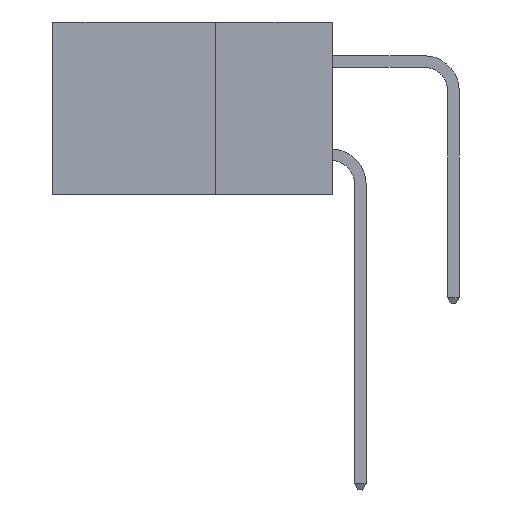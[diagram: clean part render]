
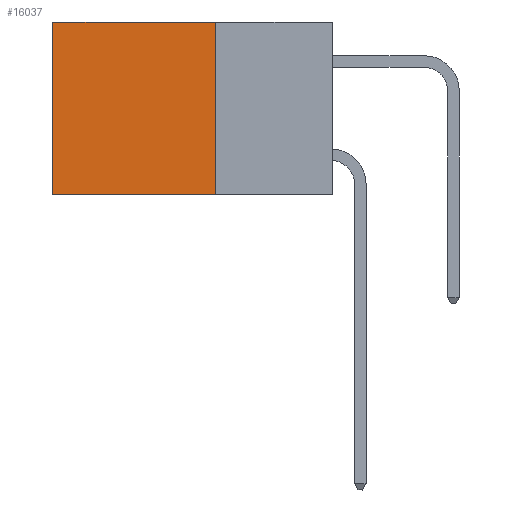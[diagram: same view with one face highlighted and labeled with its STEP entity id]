
A CAD part, left-side view. The second image highlights one B-rep face of the part: STEP entity #16037.
In plain terms, the highlighted planar face has unit normal (-1, 0, 0).
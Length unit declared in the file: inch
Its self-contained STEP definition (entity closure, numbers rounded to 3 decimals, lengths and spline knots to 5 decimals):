
#307 = ORIENTED_EDGE ( 'NONE', *, *, #5487, .T. ) ;
#901 = PLANE ( 'NONE',  #30332 ) ;
#1671 = CARTESIAN_POINT ( 'NONE',  ( 0.298, 0.6, 0. ) ) ;
#4353 = FACE_OUTER_BOUND ( 'NONE', #22903, .T. ) ;
#4789 = VECTOR ( 'NONE', #14758, 39.37008 ) ;
#5099 = VERTEX_POINT ( 'NONE', #7915 ) ;
#5487 = EDGE_CURVE ( 'NONE', #5099, #25406, #22364, .T. ) ;
#6231 = VECTOR ( 'NONE', #30755, 39.37008 ) ;
#6357 = DIRECTION ( 'NONE',  ( 0., 0., -1. ) ) ;
#6501 = CARTESIAN_POINT ( 'NONE',  ( 0.298, 0.25, 0. ) ) ;
#7915 = CARTESIAN_POINT ( 'NONE',  ( 0.298, 0.6, 0. ) ) ;
#8880 = EDGE_CURVE ( 'NONE', #11142, #5099, #28286, .T. ) ;
#9814 = ORIENTED_EDGE ( 'NONE', *, *, #23016, .F. ) ;
#10846 = VERTEX_POINT ( 'NONE', #28779 ) ;
#11142 = VERTEX_POINT ( 'NONE', #16438 ) ;
#11701 = CARTESIAN_POINT ( 'NONE',  ( 0.298, 0.25, 0. ) ) ;
#13079 = VECTOR ( 'NONE', #28653, 39.37008 ) ;
#14372 = VECTOR ( 'NONE', #18755, 39.37008 ) ;
#14758 = DIRECTION ( 'NONE',  ( 0., 0., -1. ) ) ;
#16037 = ADVANCED_FACE ( 'NONE', ( #4353 ), #901, .F. ) ;
#16438 = CARTESIAN_POINT ( 'NONE',  ( 0.298, 0.25, 0. ) ) ;
#18755 = DIRECTION ( 'NONE',  ( 0., 0., -1. ) ) ;
#19028 = CARTESIAN_POINT ( 'NONE',  ( 0.298, 0.6, -0.37 ) ) ;
#20105 = LINE ( 'NONE', #6501, #4789 ) ;
#20673 = LINE ( 'NONE', #25373, #6231 ) ;
#22364 = LINE ( 'NONE', #1671, #14372 ) ;
#22608 = DIRECTION ( 'NONE',  ( 1., 0., 0. ) ) ;
#22903 = EDGE_LOOP ( 'NONE', ( #307, #9814, #26659, #26672 ) ) ;
#23016 = EDGE_CURVE ( 'NONE', #10846, #25406, #20673, .T. ) ;
#25373 = CARTESIAN_POINT ( 'NONE',  ( 0.298, 0.25, -0.37 ) ) ;
#25406 = VERTEX_POINT ( 'NONE', #19028 ) ;
#26659 = ORIENTED_EDGE ( 'NONE', *, *, #32722, .F. ) ;
#26672 = ORIENTED_EDGE ( 'NONE', *, *, #8880, .T. ) ;
#28286 = LINE ( 'NONE', #33921, #13079 ) ;
#28653 = DIRECTION ( 'NONE',  ( 0., 1., 0. ) ) ;
#28779 = CARTESIAN_POINT ( 'NONE',  ( 0.298, 0.25, -0.37 ) ) ;
#30332 = AXIS2_PLACEMENT_3D ( 'NONE', #11701, #22608, #6357 ) ;
#30755 = DIRECTION ( 'NONE',  ( 0., 1., 0. ) ) ;
#32722 = EDGE_CURVE ( 'NONE', #11142, #10846, #20105, .T. ) ;
#33921 = CARTESIAN_POINT ( 'NONE',  ( 0.298, 0.25, 0. ) ) ;
